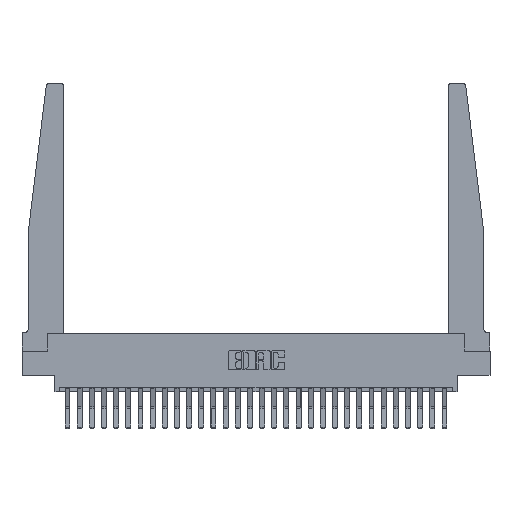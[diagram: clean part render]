
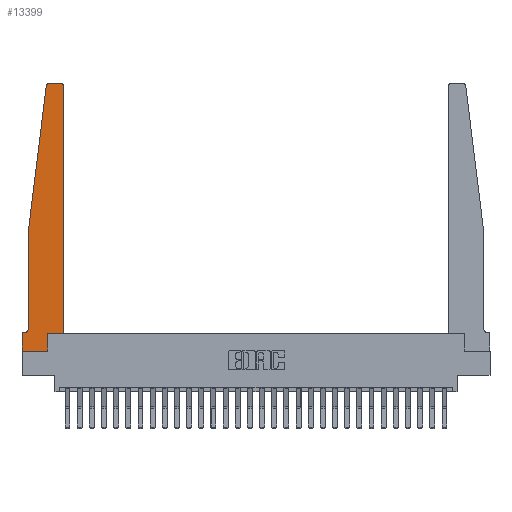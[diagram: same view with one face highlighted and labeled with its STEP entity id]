
A CAD part, top view. The second image highlights one B-rep face of the part: STEP entity #13399.
In plain terms, the highlighted planar face has unit normal (0, 0, 1).
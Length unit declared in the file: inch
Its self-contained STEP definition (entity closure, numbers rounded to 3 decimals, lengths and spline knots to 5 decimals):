
#407 = VERTEX_POINT ( 'NONE', #24516 ) ;
#635 = CARTESIAN_POINT ( 'NONE',  ( 0.27653, 2.75, 0.37 ) ) ;
#646 = EDGE_CURVE ( 'NONE', #5554, #14079, #6411, .T. ) ;
#1042 = DIRECTION ( 'NONE',  ( 0., 0., 1. ) ) ;
#1086 = LINE ( 'NONE', #24601, #1944 ) ;
#1237 = LINE ( 'NONE', #16183, #13223 ) ;
#1371 = ORIENTED_EDGE ( 'NONE', *, *, #26800, .T. ) ;
#1451 = CARTESIAN_POINT ( 'NONE',  ( 0.425, 0.18, 0.37 ) ) ;
#1586 = ORIENTED_EDGE ( 'NONE', *, *, #21061, .T. ) ;
#1944 = VECTOR ( 'NONE', #26847, 39.37008 ) ;
#2060 = ORIENTED_EDGE ( 'NONE', *, *, #3136, .T. ) ;
#2605 = VERTEX_POINT ( 'NONE', #19305 ) ;
#3134 = CARTESIAN_POINT ( 'NONE',  ( 0.015, 0.2375, 0.37 ) ) ;
#3136 = EDGE_CURVE ( 'NONE', #6389, #22402, #17577, .T. ) ;
#3140 = CARTESIAN_POINT ( 'NONE',  ( 0., 0.1875, 0.37 ) ) ;
#3470 = VECTOR ( 'NONE', #20640, 39.37008 ) ;
#3659 = CARTESIAN_POINT ( 'NONE',  ( 0.065, 1.25, 0.37 ) ) ;
#4586 = EDGE_CURVE ( 'NONE', #22402, #407, #15997, .T. ) ;
#5554 = VERTEX_POINT ( 'NONE', #23521 ) ;
#6320 = DIRECTION ( 'NONE',  ( 1., 0., 0. ) ) ;
#6389 = VERTEX_POINT ( 'NONE', #27395 ) ;
#6411 = LINE ( 'NONE', #15215, #10926 ) ;
#6570 = EDGE_LOOP ( 'NONE', ( #2060, #10531, #8564, #26462, #21476, #15328, #1371, #1586, #24579, #17529, #23134, #13555 ) ) ;
#6600 = AXIS2_PLACEMENT_3D ( 'NONE', #15042, #23312, #21214 ) ;
#6702 = CARTESIAN_POINT ( 'NONE',  ( 0.2605, 0.18, 0.37 ) ) ;
#7283 = AXIS2_PLACEMENT_3D ( 'NONE', #3134, #9558, #18084 ) ;
#7335 = EDGE_CURVE ( 'NONE', #2605, #24168, #17316, .T. ) ;
#8025 = CARTESIAN_POINT ( 'NONE',  ( 0.425, 0.18, 0.37 ) ) ;
#8469 = EDGE_CURVE ( 'NONE', #12459, #2605, #26511, .T. ) ;
#8545 = LINE ( 'NONE', #19471, #17665 ) ;
#8564 = ORIENTED_EDGE ( 'NONE', *, *, #12629, .T. ) ;
#9558 = DIRECTION ( 'NONE',  ( 0., 0., -1. ) ) ;
#10005 = CARTESIAN_POINT ( 'NONE',  ( 0.065, 1.25, 0.37 ) ) ;
#10236 = VECTOR ( 'NONE', #20930, 39.37008 ) ;
#10527 = DIRECTION ( 'NONE',  ( 0., 0., 1. ) ) ;
#10531 = ORIENTED_EDGE ( 'NONE', *, *, #4586, .T. ) ;
#10790 = DIRECTION ( 'NONE',  ( 1., 0., 0. ) ) ;
#10926 = VECTOR ( 'NONE', #13108, 39.37008 ) ;
#12348 = CARTESIAN_POINT ( 'NONE',  ( 0.425, 2.72, 0.37 ) ) ;
#12459 = VERTEX_POINT ( 'NONE', #22461 ) ;
#12629 = EDGE_CURVE ( 'NONE', #407, #15000, #20779, .T. ) ;
#12635 = LINE ( 'NONE', #16577, #10236 ) ;
#13108 = DIRECTION ( 'NONE',  ( 0., 1., 0. ) ) ;
#13223 = VECTOR ( 'NONE', #24749, 39.37008 ) ;
#13339 = VERTEX_POINT ( 'NONE', #1451 ) ;
#13399 = ADVANCED_FACE ( 'NONE', ( #22839 ), #22294, .T. ) ;
#13555 = ORIENTED_EDGE ( 'NONE', *, *, #27253, .T. ) ;
#13792 = VERTEX_POINT ( 'NONE', #22264 ) ;
#14079 = VERTEX_POINT ( 'NONE', #6702 ) ;
#14209 = DIRECTION ( 'NONE',  ( -0.122, -0.992, 0. ) ) ;
#14275 = AXIS2_PLACEMENT_3D ( 'NONE', #23129, #10527, #21298 ) ;
#14673 = EDGE_CURVE ( 'NONE', #15000, #12459, #1086, .T. ) ;
#15000 = VERTEX_POINT ( 'NONE', #3659 ) ;
#15042 = CARTESIAN_POINT ( 'NONE',  ( 0.27653, 2.72, 0.37 ) ) ;
#15215 = CARTESIAN_POINT ( 'NONE',  ( 0.2605, 0.18, 0.37 ) ) ;
#15328 = ORIENTED_EDGE ( 'NONE', *, *, #7335, .T. ) ;
#15997 = CIRCLE ( 'NONE', #6600, 0.03 ) ;
#16183 = CARTESIAN_POINT ( 'NONE',  ( 0.425, 0.18, 0.37 ) ) ;
#16577 = CARTESIAN_POINT ( 'NONE',  ( 0., 0., 0.37 ) ) ;
#17316 = LINE ( 'NONE', #25892, #18608 ) ;
#17351 = AXIS2_PLACEMENT_3D ( 'NONE', #3140, #1042, #6320 ) ;
#17378 = CARTESIAN_POINT ( 'NONE',  ( 0., 0.1875, 0.37 ) ) ;
#17388 = VECTOR ( 'NONE', #14209, 39.37008 ) ;
#17529 = ORIENTED_EDGE ( 'NONE', *, *, #25070, .T. ) ;
#17577 = LINE ( 'NONE', #17716, #21910 ) ;
#17665 = VECTOR ( 'NONE', #10790, 39.37008 ) ;
#17716 = CARTESIAN_POINT ( 'NONE',  ( 0.25, 2.75, 0.37 ) ) ;
#18084 = DIRECTION ( 'NONE',  ( -1., 0., 0. ) ) ;
#18608 = VECTOR ( 'NONE', #23771, 39.37008 ) ;
#19203 = VERTEX_POINT ( 'NONE', #12348 ) ;
#19305 = CARTESIAN_POINT ( 'NONE',  ( 0.015, 0.1875, 0.37 ) ) ;
#19471 = CARTESIAN_POINT ( 'NONE',  ( 0., 0., 0.37 ) ) ;
#20534 = CIRCLE ( 'NONE', #14275, 0.03 ) ;
#20640 = DIRECTION ( 'NONE',  ( 1., 0., 0. ) ) ;
#20779 = LINE ( 'NONE', #10005, #17388 ) ;
#20930 = DIRECTION ( 'NONE',  ( 0., -1., 0. ) ) ;
#21061 = EDGE_CURVE ( 'NONE', #13792, #5554, #8545, .T. ) ;
#21214 = DIRECTION ( 'NONE',  ( 1., 0., 0. ) ) ;
#21298 = DIRECTION ( 'NONE',  ( 1., 0., 0. ) ) ;
#21476 = ORIENTED_EDGE ( 'NONE', *, *, #8469, .T. ) ;
#21910 = VECTOR ( 'NONE', #26580, 39.37008 ) ;
#22071 = EDGE_CURVE ( 'NONE', #13339, #19203, #1237, .T. ) ;
#22264 = CARTESIAN_POINT ( 'NONE',  ( 0., 0., 0.37 ) ) ;
#22294 = PLANE ( 'NONE',  #17351 ) ;
#22402 = VERTEX_POINT ( 'NONE', #635 ) ;
#22461 = CARTESIAN_POINT ( 'NONE',  ( 0.065, 0.2375, 0.37 ) ) ;
#22839 = FACE_OUTER_BOUND ( 'NONE', #6570, .T. ) ;
#23129 = CARTESIAN_POINT ( 'NONE',  ( 0.395, 2.72, 0.37 ) ) ;
#23134 = ORIENTED_EDGE ( 'NONE', *, *, #22071, .T. ) ;
#23312 = DIRECTION ( 'NONE',  ( 0., 0., 1. ) ) ;
#23521 = CARTESIAN_POINT ( 'NONE',  ( 0.2605, 0., 0.37 ) ) ;
#23771 = DIRECTION ( 'NONE',  ( -1., 0., 0. ) ) ;
#24168 = VERTEX_POINT ( 'NONE', #17378 ) ;
#24516 = CARTESIAN_POINT ( 'NONE',  ( 0.24675, 2.72367, 0.37 ) ) ;
#24579 = ORIENTED_EDGE ( 'NONE', *, *, #646, .T. ) ;
#24601 = CARTESIAN_POINT ( 'NONE',  ( 0.065, 1.25, 0.37 ) ) ;
#24749 = DIRECTION ( 'NONE',  ( 0., 1., 0. ) ) ;
#25070 = EDGE_CURVE ( 'NONE', #14079, #13339, #27239, .T. ) ;
#25892 = CARTESIAN_POINT ( 'NONE',  ( 0.065, 0.1875, 0.37 ) ) ;
#26462 = ORIENTED_EDGE ( 'NONE', *, *, #14673, .T. ) ;
#26511 = CIRCLE ( 'NONE', #7283, 0.05 ) ;
#26580 = DIRECTION ( 'NONE',  ( -1., 0., 0. ) ) ;
#26800 = EDGE_CURVE ( 'NONE', #24168, #13792, #12635, .T. ) ;
#26847 = DIRECTION ( 'NONE',  ( 0., -1., 0. ) ) ;
#27239 = LINE ( 'NONE', #8025, #3470 ) ;
#27253 = EDGE_CURVE ( 'NONE', #19203, #6389, #20534, .T. ) ;
#27395 = CARTESIAN_POINT ( 'NONE',  ( 0.395, 2.75, 0.37 ) ) ;
